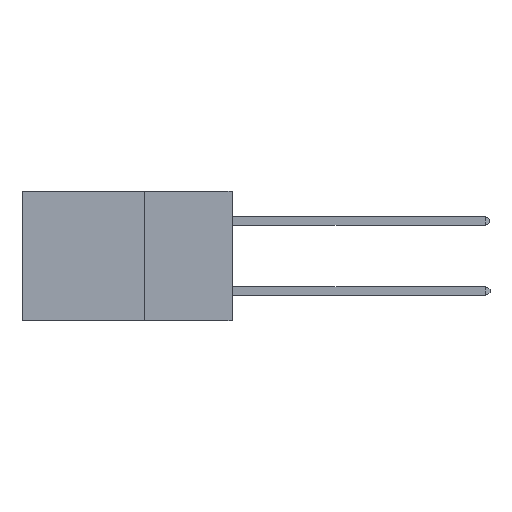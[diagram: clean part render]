
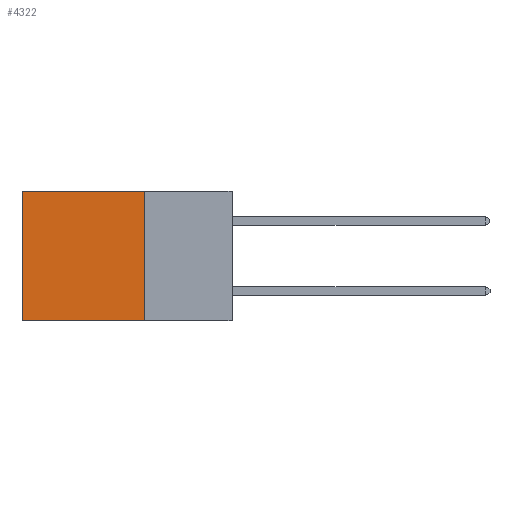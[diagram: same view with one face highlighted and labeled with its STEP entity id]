
A CAD part, left-side view. The second image highlights one B-rep face of the part: STEP entity #4322.
In plain terms, the highlighted planar face has unit normal (-1, 0, 0).
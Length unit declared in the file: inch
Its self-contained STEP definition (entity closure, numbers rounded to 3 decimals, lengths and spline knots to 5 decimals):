
#811 = ORIENTED_EDGE ( 'NONE', *, *, #5343, .T. ) ;
#1577 = DIRECTION ( 'NONE',  ( 0., 0., -1. ) ) ;
#1616 = DIRECTION ( 'NONE',  ( 0., 1., 0. ) ) ;
#2927 = VERTEX_POINT ( 'NONE', #4357 ) ;
#3118 = VECTOR ( 'NONE', #1616, 39.37008 ) ;
#3653 = FACE_OUTER_BOUND ( 'NONE', #6841, .T. ) ;
#3977 = CARTESIAN_POINT ( 'NONE',  ( 0.2875, 0.6, 0. ) ) ;
#4314 = EDGE_CURVE ( 'NONE', #11729, #7211, #6950, .T. ) ;
#4322 = ADVANCED_FACE ( 'NONE', ( #3653 ), #7250, .F. ) ;
#4357 = CARTESIAN_POINT ( 'NONE',  ( 0.2875, 0.6, 0. ) ) ;
#4401 = VECTOR ( 'NONE', #7248, 39.37008 ) ;
#4431 = CARTESIAN_POINT ( 'NONE',  ( 0.2875, 0.25, 0. ) ) ;
#4712 = LINE ( 'NONE', #3977, #11226 ) ;
#5343 = EDGE_CURVE ( 'NONE', #2927, #12575, #4712, .T. ) ;
#5675 = ORIENTED_EDGE ( 'NONE', *, *, #14634, .T. ) ;
#5847 = CARTESIAN_POINT ( 'NONE',  ( 0.2875, 0.25, -0.37 ) ) ;
#5848 = DIRECTION ( 'NONE',  ( 0., 0., -1. ) ) ;
#6442 = CARTESIAN_POINT ( 'NONE',  ( 0.2875, 0.25, 0. ) ) ;
#6841 = EDGE_LOOP ( 'NONE', ( #811, #16243, #7438, #5675 ) ) ;
#6950 = LINE ( 'NONE', #4431, #17734 ) ;
#7211 = VERTEX_POINT ( 'NONE', #11443 ) ;
#7248 = DIRECTION ( 'NONE',  ( 0., 1., 0. ) ) ;
#7250 = PLANE ( 'NONE',  #18052 ) ;
#7438 = ORIENTED_EDGE ( 'NONE', *, *, #4314, .F. ) ;
#8408 = EDGE_CURVE ( 'NONE', #7211, #12575, #11812, .T. ) ;
#8627 = CARTESIAN_POINT ( 'NONE',  ( 0.2875, 0.25, 0. ) ) ;
#8661 = CARTESIAN_POINT ( 'NONE',  ( 0.2875, 0.25, 0. ) ) ;
#10031 = DIRECTION ( 'NONE',  ( 1., 0., 0. ) ) ;
#11011 = CARTESIAN_POINT ( 'NONE',  ( 0.2875, 0.6, -0.37 ) ) ;
#11226 = VECTOR ( 'NONE', #16620, 39.37008 ) ;
#11443 = CARTESIAN_POINT ( 'NONE',  ( 0.2875, 0.25, -0.37 ) ) ;
#11729 = VERTEX_POINT ( 'NONE', #6442 ) ;
#11812 = LINE ( 'NONE', #5847, #4401 ) ;
#12575 = VERTEX_POINT ( 'NONE', #11011 ) ;
#14634 = EDGE_CURVE ( 'NONE', #11729, #2927, #17663, .T. ) ;
#16243 = ORIENTED_EDGE ( 'NONE', *, *, #8408, .F. ) ;
#16620 = DIRECTION ( 'NONE',  ( 0., 0., -1. ) ) ;
#17663 = LINE ( 'NONE', #8661, #3118 ) ;
#17734 = VECTOR ( 'NONE', #5848, 39.37008 ) ;
#18052 = AXIS2_PLACEMENT_3D ( 'NONE', #8627, #10031, #1577 ) ;
